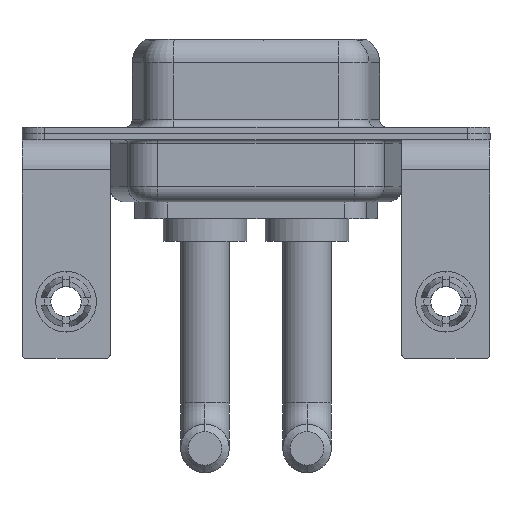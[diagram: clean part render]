
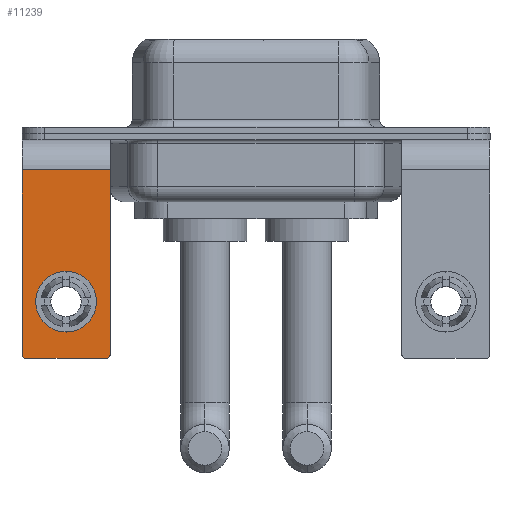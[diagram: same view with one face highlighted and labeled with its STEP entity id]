
A CAD part, front view. The second image highlights one B-rep face of the part: STEP entity #11239.
In plain terms, the highlighted planar face has unit normal (0, -1, 0).
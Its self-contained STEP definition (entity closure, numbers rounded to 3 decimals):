
#223 = AXIS2_PLACEMENT_3D ( 'NONE', #12286, #6119, #12210 ) ;
#275 = EDGE_CURVE ( 'NONE', #11388, #1366, #1937, .T. ) ;
#561 = VERTEX_POINT ( 'NONE', #1755 ) ;
#570 = VECTOR ( 'NONE', #12481, 1000. ) ;
#736 = FACE_BOUND ( 'NONE', #1785, .T. ) ;
#819 = DIRECTION ( 'NONE',  ( 0., 0., 1. ) ) ;
#1290 = EDGE_CURVE ( 'NONE', #8508, #15215, #11446, .T. ) ;
#1366 = VERTEX_POINT ( 'NONE', #11279 ) ;
#1592 = ORIENTED_EDGE ( 'NONE', *, *, #13555, .F. ) ;
#1754 = ORIENTED_EDGE ( 'NONE', *, *, #275, .T. ) ;
#1755 = CARTESIAN_POINT ( 'NONE',  ( -2.9, -6.25, -14.55 ) ) ;
#1785 = EDGE_LOOP ( 'NONE', ( #1754, #7715 ) ) ;
#1922 = DIRECTION ( 'NONE',  ( 0., 0., 1. ) ) ;
#1937 = CIRCLE ( 'NONE', #10555, 2. ) ;
#2311 = EDGE_CURVE ( 'NONE', #561, #9406, #7825, .T. ) ;
#2384 = ORIENTED_EDGE ( 'NONE', *, *, #2311, .T. ) ;
#2997 = CARTESIAN_POINT ( 'NONE',  ( 2.65, -6.25, -14.8 ) ) ;
#3417 = FACE_OUTER_BOUND ( 'NONE', #4730, .T. ) ;
#3903 = ORIENTED_EDGE ( 'NONE', *, *, #5325, .T. ) ;
#4043 = CIRCLE ( 'NONE', #11644, 2. ) ;
#4255 = ORIENTED_EDGE ( 'NONE', *, *, #1290, .T. ) ;
#4393 = VERTEX_POINT ( 'NONE', #8028 ) ;
#4396 = CARTESIAN_POINT ( 'NONE',  ( -2.65, -6.25, -14.8 ) ) ;
#4730 = EDGE_LOOP ( 'NONE', ( #8690, #2384, #14671, #3903, #1592, #4255 ) ) ;
#4737 = CARTESIAN_POINT ( 'NONE',  ( 2.9, -6.25, -14.8 ) ) ;
#4941 = CIRCLE ( 'NONE', #12281, 0.25 ) ;
#5191 = DIRECTION ( 'NONE',  ( 0., 0., -1. ) ) ;
#5325 = EDGE_CURVE ( 'NONE', #10190, #4393, #4941, .T. ) ;
#5953 = CARTESIAN_POINT ( 'NONE',  ( 0., -6.25, -11.07 ) ) ;
#6119 = DIRECTION ( 'NONE',  ( 0., -1., 0. ) ) ;
#6171 = EDGE_CURVE ( 'NONE', #15215, #561, #6808, .T. ) ;
#6755 = DIRECTION ( 'NONE',  ( 0., 1., 0. ) ) ;
#6808 = LINE ( 'NONE', #15301, #8118 ) ;
#7044 = VECTOR ( 'NONE', #14795, 1000. ) ;
#7130 = CARTESIAN_POINT ( 'NONE',  ( 2.9, -6.25, -2.4 ) ) ;
#7715 = ORIENTED_EDGE ( 'NONE', *, *, #14108, .T. ) ;
#7778 = DIRECTION ( 'NONE',  ( 0., 0., 1. ) ) ;
#7825 = CIRCLE ( 'NONE', #223, 0.25 ) ;
#8028 = CARTESIAN_POINT ( 'NONE',  ( 2.9, -6.25, -14.55 ) ) ;
#8118 = VECTOR ( 'NONE', #12888, 1000. ) ;
#8250 = DIRECTION ( 'NONE',  ( 0., 1., 0. ) ) ;
#8397 = LINE ( 'NONE', #4737, #570 ) ;
#8508 = VERTEX_POINT ( 'NONE', #7130 ) ;
#8690 = ORIENTED_EDGE ( 'NONE', *, *, #6171, .T. ) ;
#8970 = CARTESIAN_POINT ( 'NONE',  ( 0., -6.25, -11.07 ) ) ;
#9059 = CARTESIAN_POINT ( 'NONE',  ( 2.65, -6.25, -14.55 ) ) ;
#9384 = PLANE ( 'NONE',  #12428 ) ;
#9406 = VERTEX_POINT ( 'NONE', #4396 ) ;
#10190 = VERTEX_POINT ( 'NONE', #2997 ) ;
#10236 = VECTOR ( 'NONE', #5191, 1000. ) ;
#10555 = AXIS2_PLACEMENT_3D ( 'NONE', #5953, #10646, #13317 ) ;
#10643 = CARTESIAN_POINT ( 'NONE',  ( 2.9, -6.25, -2.4 ) ) ;
#10646 = DIRECTION ( 'NONE',  ( 0., 1., 0. ) ) ;
#11239 = ADVANCED_FACE ( 'NONE', ( #736, #3417 ), #9384, .F. ) ;
#11279 = CARTESIAN_POINT ( 'NONE',  ( 0., -6.25, -9.07 ) ) ;
#11388 = VERTEX_POINT ( 'NONE', #14769 ) ;
#11446 = LINE ( 'NONE', #13672, #7044 ) ;
#11644 = AXIS2_PLACEMENT_3D ( 'NONE', #8970, #6755, #7778 ) ;
#11832 = EDGE_CURVE ( 'NONE', #10190, #9406, #8397, .T. ) ;
#12210 = DIRECTION ( 'NONE',  ( 0., 0., 1. ) ) ;
#12281 = AXIS2_PLACEMENT_3D ( 'NONE', #9059, #12693, #1922 ) ;
#12286 = CARTESIAN_POINT ( 'NONE',  ( -2.65, -6.25, -14.55 ) ) ;
#12428 = AXIS2_PLACEMENT_3D ( 'NONE', #10643, #8250, #819 ) ;
#12481 = DIRECTION ( 'NONE',  ( -1., 0., 0. ) ) ;
#12557 = LINE ( 'NONE', #13690, #10236 ) ;
#12693 = DIRECTION ( 'NONE',  ( 0., -1., 0. ) ) ;
#12888 = DIRECTION ( 'NONE',  ( 0., 0., -1. ) ) ;
#12965 = CARTESIAN_POINT ( 'NONE',  ( -2.9, -6.25, -2.4 ) ) ;
#13317 = DIRECTION ( 'NONE',  ( 0., 0., 1. ) ) ;
#13555 = EDGE_CURVE ( 'NONE', #8508, #4393, #12557, .T. ) ;
#13672 = CARTESIAN_POINT ( 'NONE',  ( 2.9, -6.25, -2.4 ) ) ;
#13690 = CARTESIAN_POINT ( 'NONE',  ( 2.9, -6.25, -2.4 ) ) ;
#14108 = EDGE_CURVE ( 'NONE', #1366, #11388, #4043, .T. ) ;
#14671 = ORIENTED_EDGE ( 'NONE', *, *, #11832, .F. ) ;
#14769 = CARTESIAN_POINT ( 'NONE',  ( 0., -6.25, -13.07 ) ) ;
#14795 = DIRECTION ( 'NONE',  ( -1., 0., 0. ) ) ;
#15215 = VERTEX_POINT ( 'NONE', #12965 ) ;
#15301 = CARTESIAN_POINT ( 'NONE',  ( -2.9, -6.25, -2.4 ) ) ;
